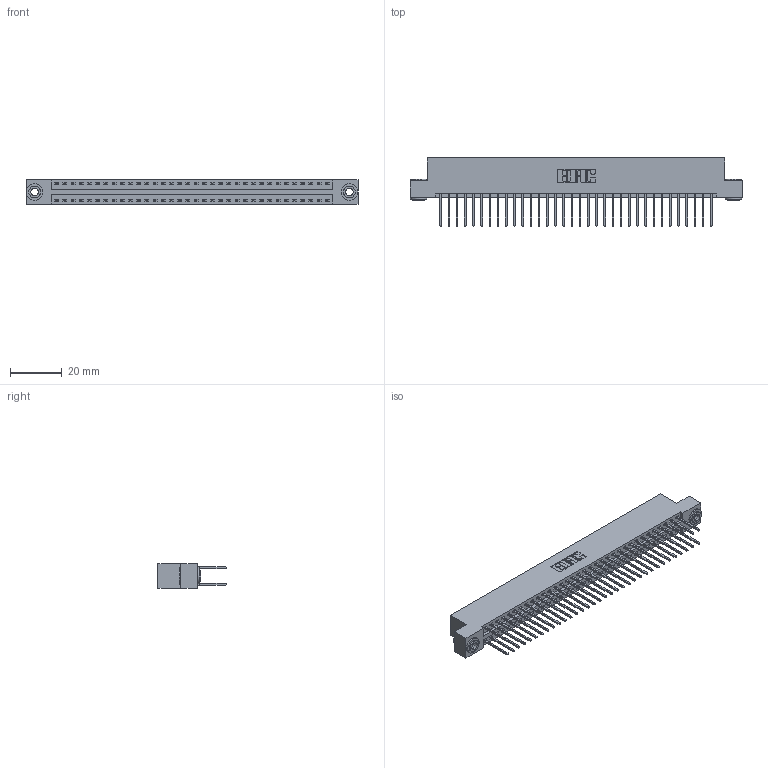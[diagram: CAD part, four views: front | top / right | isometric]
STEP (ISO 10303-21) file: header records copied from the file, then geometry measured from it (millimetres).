
FILE_DESCRIPTION (( 'STEP AP203' ), '1' );
FILE_NAME ('346-068-522-203.STEP', '2022-05-24T18:55:45', ( '' ), ( '' ), 'SwSTEP 2.0', 'SolidWorks 2020', '' );
FILE_SCHEMA (( 'CONFIG_CONTROL_DESIGN' ));
Length unit declared in the file: inch
Products named in the file (4): 345-250-002_345-250-002-102; 345-292-001_345-293-122; 346 Part_Flush Mounting Lugs - 0.156 Dia-TH; 346-068-522-203
Assembly tree (71 placements, depth 2):
  346-068-522-203
    346 Part_Flush Mounting Lugs - 0.156 Dia-TH
    345-292-001_345-293-122  x68
    345-250-002_345-250-002-102  x2
Bounding box: 128.52 x 26.42 x 9.4 mm (x, y, z)
Volume: 12646.1 mm3; surface area: 18313.6 mm2
Topology: 71 solids, 71 shells, 3710 faces, 10981 edges, 7226 vertices
Faces by surface type: plane 2480, cylinder 1222, cone 8
Entity records: 24350 total; most frequent: CARTESIAN_POINT 4005, ORIENTED_EDGE 3930, DIRECTION 3611, EDGE_CURVE 1965, VECTOR 1673, LINE 1673, VERTEX_POINT 1306, AXIS2_PLACEMENT_3D 969
